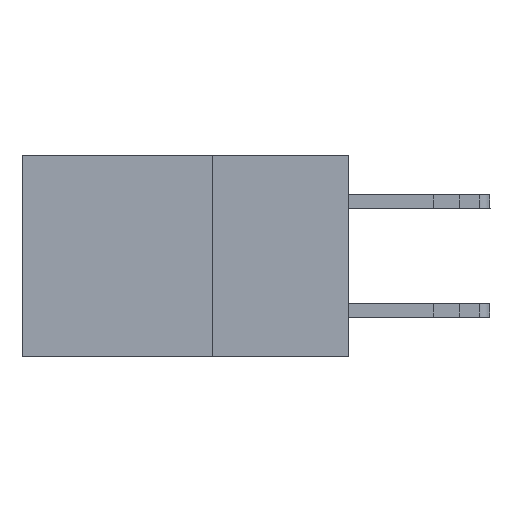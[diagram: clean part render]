
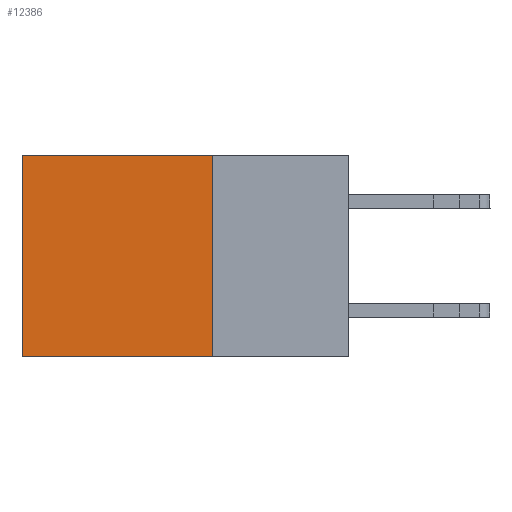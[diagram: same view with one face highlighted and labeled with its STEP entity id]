
A CAD part, left-side view. The second image highlights one B-rep face of the part: STEP entity #12386.
In plain terms, the highlighted planar face has unit normal (-1, 0, 0).
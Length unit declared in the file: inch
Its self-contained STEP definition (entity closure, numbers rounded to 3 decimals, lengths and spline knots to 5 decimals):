
#197 = VERTEX_POINT ( 'NONE', #10646 ) ;
#733 = ORIENTED_EDGE ( 'NONE', *, *, #10354, .T. ) ;
#1314 = DIRECTION ( 'NONE',  ( 1., 0., 0. ) ) ;
#1640 = LINE ( 'NONE', #10037, #1999 ) ;
#1913 = CARTESIAN_POINT ( 'NONE',  ( 0.2615, 0.6, 0. ) ) ;
#1999 = VECTOR ( 'NONE', #5965, 39.37008 ) ;
#2229 = FACE_OUTER_BOUND ( 'NONE', #6541, .T. ) ;
#2427 = DIRECTION ( 'NONE',  ( 0., 0., -1. ) ) ;
#2752 = EDGE_CURVE ( 'NONE', #6965, #3494, #5759, .T. ) ;
#2826 = VECTOR ( 'NONE', #7848, 39.37008 ) ;
#3039 = ORIENTED_EDGE ( 'NONE', *, *, #2752, .F. ) ;
#3220 = EDGE_CURVE ( 'NONE', #5142, #3494, #6862, .T. ) ;
#3327 = CARTESIAN_POINT ( 'NONE',  ( 0.2615, 0.25, -0.37 ) ) ;
#3479 = CARTESIAN_POINT ( 'NONE',  ( 0.2615, 0.6, -0.37 ) ) ;
#3494 = VERTEX_POINT ( 'NONE', #7277 ) ;
#4416 = AXIS2_PLACEMENT_3D ( 'NONE', #3327, #1314, #2427 ) ;
#4725 = DIRECTION ( 'NONE',  ( 0., 1., 0. ) ) ;
#5142 = VERTEX_POINT ( 'NONE', #1913 ) ;
#5171 = DIRECTION ( 'NONE',  ( 0., 0., -1. ) ) ;
#5759 = LINE ( 'NONE', #7934, #7008 ) ;
#5965 = DIRECTION ( 'NONE',  ( 0., 1., 0. ) ) ;
#6272 = CARTESIAN_POINT ( 'NONE',  ( 0.2615, 0.25, -0.37 ) ) ;
#6502 = PLANE ( 'NONE',  #4416 ) ;
#6541 = EDGE_LOOP ( 'NONE', ( #13579, #3039, #9134, #733 ) ) ;
#6862 = LINE ( 'NONE', #3479, #2826 ) ;
#6965 = VERTEX_POINT ( 'NONE', #10374 ) ;
#7008 = VECTOR ( 'NONE', #4725, 39.37008 ) ;
#7277 = CARTESIAN_POINT ( 'NONE',  ( 0.2615, 0.6, -0.37 ) ) ;
#7848 = DIRECTION ( 'NONE',  ( 0., 0., -1. ) ) ;
#7934 = CARTESIAN_POINT ( 'NONE',  ( 0.2615, 0.25, -0.37 ) ) ;
#8828 = VECTOR ( 'NONE', #5171, 39.37008 ) ;
#9134 = ORIENTED_EDGE ( 'NONE', *, *, #9650, .F. ) ;
#9650 = EDGE_CURVE ( 'NONE', #197, #6965, #13698, .T. ) ;
#10037 = CARTESIAN_POINT ( 'NONE',  ( 0.2615, 0.25, 0. ) ) ;
#10354 = EDGE_CURVE ( 'NONE', #197, #5142, #1640, .T. ) ;
#10374 = CARTESIAN_POINT ( 'NONE',  ( 0.2615, 0.25, -0.37 ) ) ;
#10646 = CARTESIAN_POINT ( 'NONE',  ( 0.2615, 0.25, 0. ) ) ;
#12386 = ADVANCED_FACE ( 'NONE', ( #2229 ), #6502, .F. ) ;
#13579 = ORIENTED_EDGE ( 'NONE', *, *, #3220, .T. ) ;
#13698 = LINE ( 'NONE', #6272, #8828 ) ;
